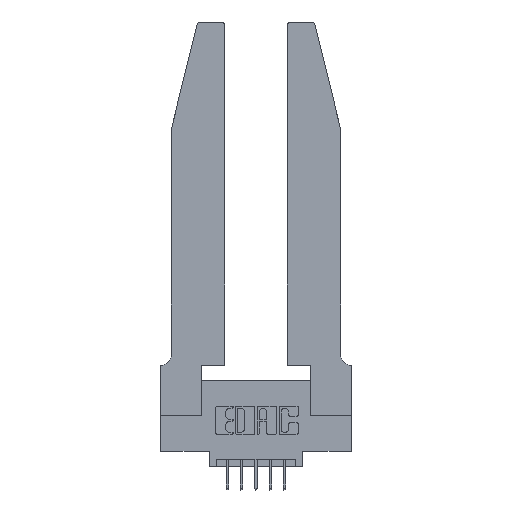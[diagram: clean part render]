
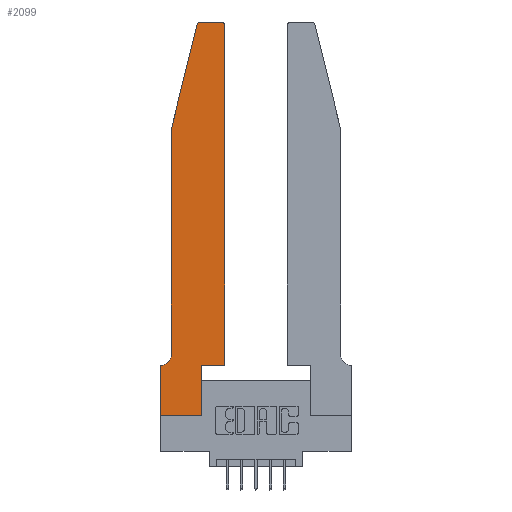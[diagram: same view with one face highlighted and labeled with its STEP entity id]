
A CAD part, top view. The second image highlights one B-rep face of the part: STEP entity #2099.
In plain terms, the highlighted planar face has unit normal (0, 0, 1).
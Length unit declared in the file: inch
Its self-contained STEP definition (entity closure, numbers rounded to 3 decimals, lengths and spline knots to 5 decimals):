
#158 = CARTESIAN_POINT ( 'NONE',  ( 0.4505, 2.72, 0.37 ) ) ;
#304 = CARTESIAN_POINT ( 'NONE',  ( 0.4505, 0.35, 0.37 ) ) ;
#344 = CARTESIAN_POINT ( 'NONE',  ( 0.0755, 0.35, 0.37 ) ) ;
#352 = DIRECTION ( 'NONE',  ( 1., 0., 0. ) ) ;
#441 = EDGE_LOOP ( 'NONE', ( #3815, #9339, #12684, #7198, #11484, #3591, #2349, #11293, #7608, #2999, #10206, #9106 ) ) ;
#675 = CARTESIAN_POINT ( 'NONE',  ( 0.4205, 2.72, 0.37 ) ) ;
#693 = CARTESIAN_POINT ( 'NONE',  ( 0., 0., 0.37 ) ) ;
#889 = VERTEX_POINT ( 'NONE', #12933 ) ;
#914 = VERTEX_POINT ( 'NONE', #158 ) ;
#1058 = AXIS2_PLACEMENT_3D ( 'NONE', #675, #5839, #12461 ) ;
#1292 = VECTOR ( 'NONE', #4084, 39.37008 ) ;
#1444 = EDGE_CURVE ( 'NONE', #1683, #10851, #10635, .T. ) ;
#1453 = DIRECTION ( 'NONE',  ( 1., 0., 0. ) ) ;
#1557 = CARTESIAN_POINT ( 'NONE',  ( 0.0755, 2., 0.37 ) ) ;
#1683 = VERTEX_POINT ( 'NONE', #8340 ) ;
#1837 = CARTESIAN_POINT ( 'NONE',  ( 0.4505, 0.35, 0.37 ) ) ;
#1891 = VECTOR ( 'NONE', #7796, 39.37008 ) ;
#2099 = ADVANCED_FACE ( 'NONE', ( #4047 ), #4747, .T. ) ;
#2105 = CARTESIAN_POINT ( 'NONE',  ( 0.0755, 2., 0.37 ) ) ;
#2247 = DIRECTION ( 'NONE',  ( -0.239, -0.971, 0. ) ) ;
#2349 = ORIENTED_EDGE ( 'NONE', *, *, #6718, .T. ) ;
#2474 = EDGE_CURVE ( 'NONE', #10851, #8104, #11602, .T. ) ;
#2999 = ORIENTED_EDGE ( 'NONE', *, *, #12152, .T. ) ;
#3058 = VECTOR ( 'NONE', #2247, 39.37008 ) ;
#3222 = CARTESIAN_POINT ( 'NONE',  ( 0.2865, 0.35, 0.37 ) ) ;
#3556 = DIRECTION ( 'NONE',  ( -1., 0., 0. ) ) ;
#3591 = ORIENTED_EDGE ( 'NONE', *, *, #11168, .T. ) ;
#3594 = EDGE_CURVE ( 'NONE', #13707, #11148, #9718, .T. ) ;
#3815 = ORIENTED_EDGE ( 'NONE', *, *, #5913, .T. ) ;
#4047 = FACE_OUTER_BOUND ( 'NONE', #441, .T. ) ;
#4084 = DIRECTION ( 'NONE',  ( 0., -1., 0. ) ) ;
#4168 = DIRECTION ( 'NONE',  ( 0., -1., 0. ) ) ;
#4353 = CIRCLE ( 'NONE', #12808, 0.07 ) ;
#4747 = PLANE ( 'NONE',  #9735 ) ;
#5082 = CARTESIAN_POINT ( 'NONE',  ( 0.25487, 2.72718, 0.37 ) ) ;
#5190 = VERTEX_POINT ( 'NONE', #693 ) ;
#5214 = CIRCLE ( 'NONE', #1058, 0.03 ) ;
#5218 = CARTESIAN_POINT ( 'NONE',  ( 0.2605, 2.75, 0.37 ) ) ;
#5839 = DIRECTION ( 'NONE',  ( 0., 0., 1. ) ) ;
#5844 = LINE ( 'NONE', #5218, #6367 ) ;
#5913 = EDGE_CURVE ( 'NONE', #9802, #1683, #5844, .T. ) ;
#6051 = CARTESIAN_POINT ( 'NONE',  ( 0.4505, 0.35, 0.37 ) ) ;
#6212 = VECTOR ( 'NONE', #352, 39.37008 ) ;
#6286 = DIRECTION ( 'NONE',  ( 0., 1., 0. ) ) ;
#6367 = VECTOR ( 'NONE', #7509, 39.37008 ) ;
#6412 = CARTESIAN_POINT ( 'NONE',  ( 0., 0., 0.37 ) ) ;
#6676 = VECTOR ( 'NONE', #6286, 39.37008 ) ;
#6718 = EDGE_CURVE ( 'NONE', #12154, #5190, #11223, .T. ) ;
#7090 = AXIS2_PLACEMENT_3D ( 'NONE', #7834, #8957, #1453 ) ;
#7198 = ORIENTED_EDGE ( 'NONE', *, *, #9097, .T. ) ;
#7265 = CARTESIAN_POINT ( 'NONE',  ( 0.0755, 2., 0.37 ) ) ;
#7491 = CARTESIAN_POINT ( 'NONE',  ( 0.4205, 2.75, 0.37 ) ) ;
#7509 = DIRECTION ( 'NONE',  ( -1., 0., 0. ) ) ;
#7608 = ORIENTED_EDGE ( 'NONE', *, *, #3594, .T. ) ;
#7693 = VERTEX_POINT ( 'NONE', #9342 ) ;
#7796 = DIRECTION ( 'NONE',  ( -1., 0., 0. ) ) ;
#7799 = LINE ( 'NONE', #7265, #1292 ) ;
#7834 = CARTESIAN_POINT ( 'NONE',  ( 0.284, 2.72, 0.37 ) ) ;
#7884 = LINE ( 'NONE', #1837, #11943 ) ;
#7894 = CARTESIAN_POINT ( 'NONE',  ( 0., 0.35, 0.37 ) ) ;
#7984 = DIRECTION ( 'NONE',  ( 0., 0., 1. ) ) ;
#8104 = VERTEX_POINT ( 'NONE', #1557 ) ;
#8199 = CARTESIAN_POINT ( 'NONE',  ( 0.0055, 0.42, 0.37 ) ) ;
#8340 = CARTESIAN_POINT ( 'NONE',  ( 0.284, 2.75, 0.37 ) ) ;
#8957 = DIRECTION ( 'NONE',  ( 0., 0., 1. ) ) ;
#9046 = LINE ( 'NONE', #304, #6212 ) ;
#9058 = VECTOR ( 'NONE', #13703, 39.37008 ) ;
#9097 = EDGE_CURVE ( 'NONE', #8104, #7693, #7799, .T. ) ;
#9106 = ORIENTED_EDGE ( 'NONE', *, *, #12970, .T. ) ;
#9265 = LINE ( 'NONE', #344, #1891 ) ;
#9339 = ORIENTED_EDGE ( 'NONE', *, *, #1444, .T. ) ;
#9342 = CARTESIAN_POINT ( 'NONE',  ( 0.0755, 0.42, 0.37 ) ) ;
#9418 = CARTESIAN_POINT ( 'NONE',  ( 0., 0., 0.37 ) ) ;
#9561 = CARTESIAN_POINT ( 'NONE',  ( 0.2865, 0.35, 0.37 ) ) ;
#9718 = LINE ( 'NONE', #3222, #6676 ) ;
#9735 = AXIS2_PLACEMENT_3D ( 'NONE', #7894, #7984, #10150 ) ;
#9802 = VERTEX_POINT ( 'NONE', #7491 ) ;
#9937 = CARTESIAN_POINT ( 'NONE',  ( 0., 0.35, 0.37 ) ) ;
#10101 = VERTEX_POINT ( 'NONE', #6051 ) ;
#10150 = DIRECTION ( 'NONE',  ( 1., 0., 0. ) ) ;
#10206 = ORIENTED_EDGE ( 'NONE', *, *, #12285, .T. ) ;
#10344 = DIRECTION ( 'NONE',  ( 0., 0., -1. ) ) ;
#10502 = CARTESIAN_POINT ( 'NONE',  ( 0.2865, 0., 0.37 ) ) ;
#10635 = CIRCLE ( 'NONE', #7090, 0.03 ) ;
#10851 = VERTEX_POINT ( 'NONE', #5082 ) ;
#10937 = LINE ( 'NONE', #9418, #9058 ) ;
#11148 = VERTEX_POINT ( 'NONE', #9561 ) ;
#11168 = EDGE_CURVE ( 'NONE', #889, #12154, #9265, .T. ) ;
#11223 = LINE ( 'NONE', #6412, #13569 ) ;
#11293 = ORIENTED_EDGE ( 'NONE', *, *, #12990, .T. ) ;
#11406 = DIRECTION ( 'NONE',  ( 0., 1., 0. ) ) ;
#11484 = ORIENTED_EDGE ( 'NONE', *, *, #13460, .T. ) ;
#11602 = LINE ( 'NONE', #2105, #3058 ) ;
#11943 = VECTOR ( 'NONE', #11406, 39.37008 ) ;
#12152 = EDGE_CURVE ( 'NONE', #11148, #10101, #9046, .T. ) ;
#12154 = VERTEX_POINT ( 'NONE', #9937 ) ;
#12285 = EDGE_CURVE ( 'NONE', #10101, #914, #7884, .T. ) ;
#12461 = DIRECTION ( 'NONE',  ( 1., 0., 0. ) ) ;
#12684 = ORIENTED_EDGE ( 'NONE', *, *, #2474, .T. ) ;
#12808 = AXIS2_PLACEMENT_3D ( 'NONE', #8199, #10344, #3556 ) ;
#12933 = CARTESIAN_POINT ( 'NONE',  ( 0.0055, 0.35, 0.37 ) ) ;
#12970 = EDGE_CURVE ( 'NONE', #914, #9802, #5214, .T. ) ;
#12990 = EDGE_CURVE ( 'NONE', #5190, #13707, #10937, .T. ) ;
#13460 = EDGE_CURVE ( 'NONE', #7693, #889, #4353, .T. ) ;
#13569 = VECTOR ( 'NONE', #4168, 39.37008 ) ;
#13703 = DIRECTION ( 'NONE',  ( 1., 0., 0. ) ) ;
#13707 = VERTEX_POINT ( 'NONE', #10502 ) ;
